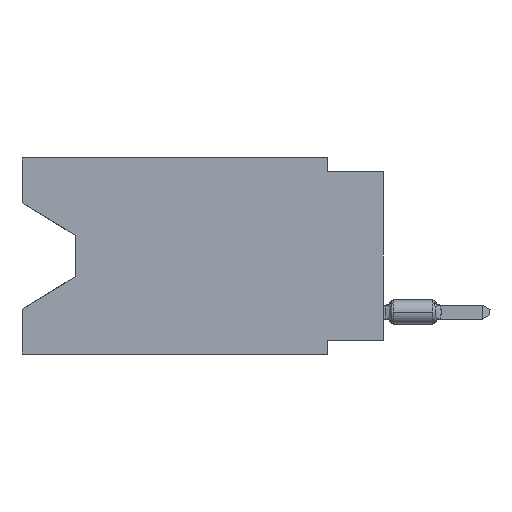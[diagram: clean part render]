
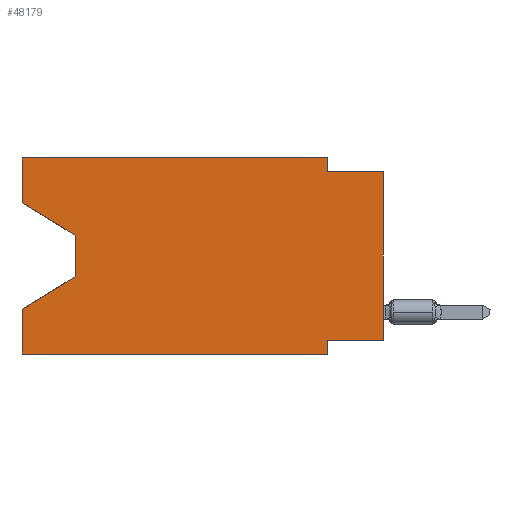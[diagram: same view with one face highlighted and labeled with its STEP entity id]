
A CAD part, left-side view. The second image highlights one B-rep face of the part: STEP entity #48179.
In plain terms, the highlighted planar face has unit normal (-1, 0, 0).
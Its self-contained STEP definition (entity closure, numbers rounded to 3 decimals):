
#1212 = CARTESIAN_POINT ( 'NONE',  ( 0., 2.54, -8.89 ) ) ;
#1379 = VECTOR ( 'NONE', #17113, 1000. ) ;
#2625 = VERTEX_POINT ( 'NONE', #46765 ) ;
#3121 = EDGE_CURVE ( 'NONE', #21638, #69854, #31625, .T. ) ;
#4730 = CARTESIAN_POINT ( 'NONE',  ( 0., 2.54, 0. ) ) ;
#4755 = VERTEX_POINT ( 'NONE', #58985 ) ;
#5147 = LINE ( 'NONE', #42364, #25742 ) ;
#5416 = VERTEX_POINT ( 'NONE', #1212 ) ;
#5901 = ORIENTED_EDGE ( 'NONE', *, *, #65146, .F. ) ;
#6545 = CARTESIAN_POINT ( 'NONE',  ( 0., 2.54, -8.255 ) ) ;
#6927 = CARTESIAN_POINT ( 'NONE',  ( 0., 13.97, -3.505 ) ) ;
#7607 = DIRECTION ( 'NONE',  ( 0., 0., -1. ) ) ;
#9766 = LINE ( 'NONE', #31231, #52641 ) ;
#10774 = LINE ( 'NONE', #48323, #31114 ) ;
#11010 = VERTEX_POINT ( 'NONE', #69037 ) ;
#12934 = LINE ( 'NONE', #34745, #52272 ) ;
#13609 = EDGE_CURVE ( 'NONE', #47972, #2625, #36363, .T. ) ;
#14532 = EDGE_CURVE ( 'NONE', #17413, #47972, #9766, .T. ) ;
#14684 = VECTOR ( 'NONE', #67998, 1000. ) ;
#16067 = VERTEX_POINT ( 'NONE', #45067 ) ;
#16148 = DIRECTION ( 'NONE',  ( 0., 1., 0. ) ) ;
#16385 = LINE ( 'NONE', #54290, #60435 ) ;
#17113 = DIRECTION ( 'NONE',  ( 0., -1., 0. ) ) ;
#17413 = VERTEX_POINT ( 'NONE', #58123 ) ;
#18378 = ORIENTED_EDGE ( 'NONE', *, *, #64464, .F. ) ;
#18735 = EDGE_CURVE ( 'NONE', #17413, #11010, #53829, .T. ) ;
#19336 = CARTESIAN_POINT ( 'NONE',  ( 0., 16.383, 0. ) ) ;
#19366 = ORIENTED_EDGE ( 'NONE', *, *, #49585, .F. ) ;
#19728 = LINE ( 'NONE', #46193, #14684 ) ;
#20035 = LINE ( 'NONE', #19336, #25054 ) ;
#20638 = DIRECTION ( 'NONE',  ( 0., 0., -1. ) ) ;
#21638 = VERTEX_POINT ( 'NONE', #4730 ) ;
#24694 = DIRECTION ( 'NONE',  ( 0., -1., 0. ) ) ;
#25054 = VECTOR ( 'NONE', #24694, 1000. ) ;
#25742 = VECTOR ( 'NONE', #47728, 1000. ) ;
#26775 = ORIENTED_EDGE ( 'NONE', *, *, #14532, .T. ) ;
#27821 = DIRECTION ( 'NONE',  ( 0., 0., 1. ) ) ;
#27844 = CARTESIAN_POINT ( 'NONE',  ( 0., 16.383, -8.89 ) ) ;
#29051 = VERTEX_POINT ( 'NONE', #68591 ) ;
#29080 = CARTESIAN_POINT ( 'NONE',  ( 0., 2.54, -8.89 ) ) ;
#29431 = DIRECTION ( 'NONE',  ( 1., 0., 0. ) ) ;
#30198 = ORIENTED_EDGE ( 'NONE', *, *, #51888, .F. ) ;
#30665 = VECTOR ( 'NONE', #20638, 1000. ) ;
#31114 = VECTOR ( 'NONE', #16148, 1000. ) ;
#31231 = CARTESIAN_POINT ( 'NONE',  ( 0., 16.383, -2.038 ) ) ;
#31473 = EDGE_CURVE ( 'NONE', #4755, #46121, #5147, .T. ) ;
#31625 = LINE ( 'NONE', #49157, #37626 ) ;
#32067 = LINE ( 'NONE', #29080, #40339 ) ;
#32518 = CARTESIAN_POINT ( 'NONE',  ( 0., 0., -0.635 ) ) ;
#34745 = CARTESIAN_POINT ( 'NONE',  ( 0., 0., -0.635 ) ) ;
#34795 = PLANE ( 'NONE',  #45731 ) ;
#34837 = CARTESIAN_POINT ( 'NONE',  ( 0., 16.383, 0. ) ) ;
#35746 = EDGE_CURVE ( 'NONE', #11010, #21638, #20035, .T. ) ;
#36363 = LINE ( 'NONE', #37799, #30665 ) ;
#37626 = VECTOR ( 'NONE', #65235, 1000. ) ;
#37799 = CARTESIAN_POINT ( 'NONE',  ( 0., 13.97, -3.505 ) ) ;
#38562 = LINE ( 'NONE', #27844, #1379 ) ;
#39822 = CARTESIAN_POINT ( 'NONE',  ( 0., 16.383, 0. ) ) ;
#40141 = ORIENTED_EDGE ( 'NONE', *, *, #13609, .T. ) ;
#40339 = VECTOR ( 'NONE', #50890, 1000. ) ;
#40539 = EDGE_LOOP ( 'NONE', ( #26775, #40141, #43565, #5901, #53490, #19366, #30198, #44553, #18378, #48287, #61797, #65665 ) ) ;
#41958 = DIRECTION ( 'NONE',  ( 0., -0.855, -0.519 ) ) ;
#42364 = CARTESIAN_POINT ( 'NONE',  ( 0., 0., 0. ) ) ;
#43565 = ORIENTED_EDGE ( 'NONE', *, *, #58204, .T. ) ;
#44553 = ORIENTED_EDGE ( 'NONE', *, *, #31473, .T. ) ;
#45067 = CARTESIAN_POINT ( 'NONE',  ( 0., 16.383, -6.852 ) ) ;
#45731 = AXIS2_PLACEMENT_3D ( 'NONE', #39822, #29431, #7607 ) ;
#45994 = VECTOR ( 'NONE', #50253, 1000. ) ;
#46121 = VERTEX_POINT ( 'NONE', #32518 ) ;
#46193 = CARTESIAN_POINT ( 'NONE',  ( 0., 13.97, -5.385 ) ) ;
#46765 = CARTESIAN_POINT ( 'NONE',  ( 0., 13.97, -5.385 ) ) ;
#47728 = DIRECTION ( 'NONE',  ( 0., 0., 1. ) ) ;
#47972 = VERTEX_POINT ( 'NONE', #6927 ) ;
#48179 = ADVANCED_FACE ( 'NONE', ( #58615 ), #34795, .F. ) ;
#48287 = ORIENTED_EDGE ( 'NONE', *, *, #3121, .F. ) ;
#48323 = CARTESIAN_POINT ( 'NONE',  ( 0., 0., -8.255 ) ) ;
#49157 = CARTESIAN_POINT ( 'NONE',  ( 0., 2.54, 0. ) ) ;
#49585 = EDGE_CURVE ( 'NONE', #62267, #5416, #32067, .T. ) ;
#50253 = DIRECTION ( 'NONE',  ( 0., 0., 1. ) ) ;
#50890 = DIRECTION ( 'NONE',  ( 0., 0., -1. ) ) ;
#51097 = EDGE_CURVE ( 'NONE', #29051, #5416, #38562, .T. ) ;
#51200 = DIRECTION ( 'NONE',  ( 0., -1., 0. ) ) ;
#51888 = EDGE_CURVE ( 'NONE', #4755, #62267, #10774, .T. ) ;
#52272 = VECTOR ( 'NONE', #51200, 1000. ) ;
#52641 = VECTOR ( 'NONE', #41958, 1000. ) ;
#53490 = ORIENTED_EDGE ( 'NONE', *, *, #51097, .T. ) ;
#53829 = LINE ( 'NONE', #34837, #45994 ) ;
#54290 = CARTESIAN_POINT ( 'NONE',  ( 0., 16.383, 0. ) ) ;
#58123 = CARTESIAN_POINT ( 'NONE',  ( 0., 16.383, -2.038 ) ) ;
#58204 = EDGE_CURVE ( 'NONE', #2625, #16067, #19728, .T. ) ;
#58615 = FACE_OUTER_BOUND ( 'NONE', #40539, .T. ) ;
#58985 = CARTESIAN_POINT ( 'NONE',  ( 0., 0., -8.255 ) ) ;
#60435 = VECTOR ( 'NONE', #27821, 1000. ) ;
#61797 = ORIENTED_EDGE ( 'NONE', *, *, #35746, .F. ) ;
#62267 = VERTEX_POINT ( 'NONE', #6545 ) ;
#63260 = CARTESIAN_POINT ( 'NONE',  ( 0., 2.54, -0.635 ) ) ;
#64464 = EDGE_CURVE ( 'NONE', #69854, #46121, #12934, .T. ) ;
#65146 = EDGE_CURVE ( 'NONE', #29051, #16067, #16385, .T. ) ;
#65235 = DIRECTION ( 'NONE',  ( 0., 0., -1. ) ) ;
#65665 = ORIENTED_EDGE ( 'NONE', *, *, #18735, .F. ) ;
#67998 = DIRECTION ( 'NONE',  ( 0., 0.855, -0.519 ) ) ;
#68591 = CARTESIAN_POINT ( 'NONE',  ( 0., 16.383, -8.89 ) ) ;
#69037 = CARTESIAN_POINT ( 'NONE',  ( 0., 16.383, 0. ) ) ;
#69854 = VERTEX_POINT ( 'NONE', #63260 ) ;
